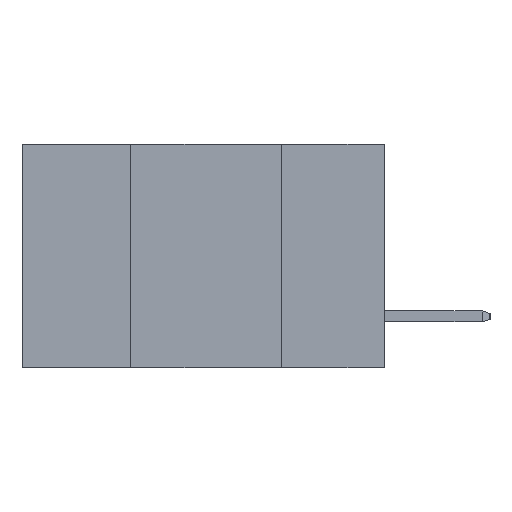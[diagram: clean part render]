
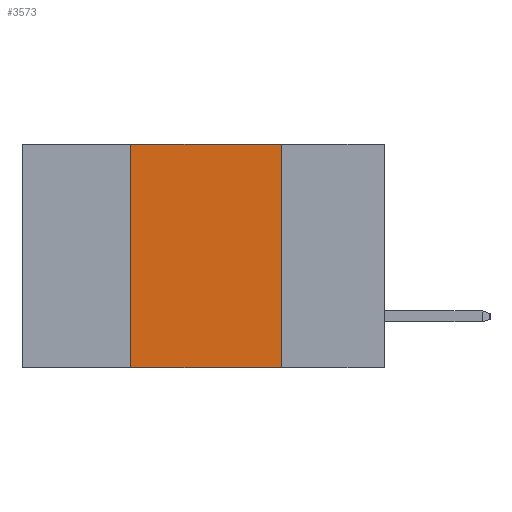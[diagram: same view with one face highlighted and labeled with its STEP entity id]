
A CAD part, left-side view. The second image highlights one B-rep face of the part: STEP entity #3573.
In plain terms, the highlighted planar face has unit normal (-1, 0, 0).
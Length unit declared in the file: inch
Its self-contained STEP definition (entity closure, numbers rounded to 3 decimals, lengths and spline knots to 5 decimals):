
#223 = CARTESIAN_POINT ( 'NONE',  ( 0., 0.17, -0.37 ) ) ;
#237 = DIRECTION ( 'NONE',  ( 0., 0., -1. ) ) ;
#474 = VERTEX_POINT ( 'NONE', #8490 ) ;
#657 = DIRECTION ( 'NONE',  ( 0., 0., -1. ) ) ;
#659 = DIRECTION ( 'NONE',  ( 1., 0., 0. ) ) ;
#681 = CARTESIAN_POINT ( 'NONE',  ( 0., 0.6, 0. ) ) ;
#688 = EDGE_CURVE ( 'NONE', #7467, #4255, #3517, .T. ) ;
#696 = PLANE ( 'NONE',  #9963 ) ;
#970 = ORIENTED_EDGE ( 'NONE', *, *, #688, .F. ) ;
#1250 = ORIENTED_EDGE ( 'NONE', *, *, #5815, .T. ) ;
#3037 = ORIENTED_EDGE ( 'NONE', *, *, #3652, .F. ) ;
#3427 = VECTOR ( 'NONE', #8375, 39.37008 ) ;
#3517 = LINE ( 'NONE', #4191, #9834 ) ;
#3573 = ADVANCED_FACE ( 'NONE', ( #9246 ), #696, .F. ) ;
#3652 = EDGE_CURVE ( 'NONE', #4255, #9063, #10945, .T. ) ;
#3735 = CARTESIAN_POINT ( 'NONE',  ( 0., 0.6, -0.37 ) ) ;
#3870 = VECTOR ( 'NONE', #237, 39.37008 ) ;
#4124 = DIRECTION ( 'NONE',  ( 0., -1., 0. ) ) ;
#4191 = CARTESIAN_POINT ( 'NONE',  ( 0., 0.6, 0. ) ) ;
#4255 = VERTEX_POINT ( 'NONE', #6121 ) ;
#5605 = ORIENTED_EDGE ( 'NONE', *, *, #8676, .F. ) ;
#5815 = EDGE_CURVE ( 'NONE', #474, #9063, #10322, .T. ) ;
#6121 = CARTESIAN_POINT ( 'NONE',  ( 0., 0.17, 0. ) ) ;
#6871 = CARTESIAN_POINT ( 'NONE',  ( 0., 0.42, 0. ) ) ;
#7221 = CARTESIAN_POINT ( 'NONE',  ( 0., 0.17, -0.37 ) ) ;
#7467 = VERTEX_POINT ( 'NONE', #6871 ) ;
#7518 = CARTESIAN_POINT ( 'NONE',  ( 0., 0.42, -0.37 ) ) ;
#8074 = VECTOR ( 'NONE', #10580, 39.37008 ) ;
#8284 = LINE ( 'NONE', #7518, #3427 ) ;
#8375 = DIRECTION ( 'NONE',  ( 0., 0., 1. ) ) ;
#8490 = CARTESIAN_POINT ( 'NONE',  ( 0., 0.42, -0.37 ) ) ;
#8676 = EDGE_CURVE ( 'NONE', #474, #7467, #8284, .T. ) ;
#9024 = EDGE_LOOP ( 'NONE', ( #3037, #970, #5605, #1250 ) ) ;
#9063 = VERTEX_POINT ( 'NONE', #7221 ) ;
#9246 = FACE_OUTER_BOUND ( 'NONE', #9024, .T. ) ;
#9834 = VECTOR ( 'NONE', #4124, 39.37008 ) ;
#9963 = AXIS2_PLACEMENT_3D ( 'NONE', #681, #659, #657 ) ;
#10322 = LINE ( 'NONE', #3735, #8074 ) ;
#10580 = DIRECTION ( 'NONE',  ( 0., -1., 0. ) ) ;
#10945 = LINE ( 'NONE', #223, #3870 ) ;
